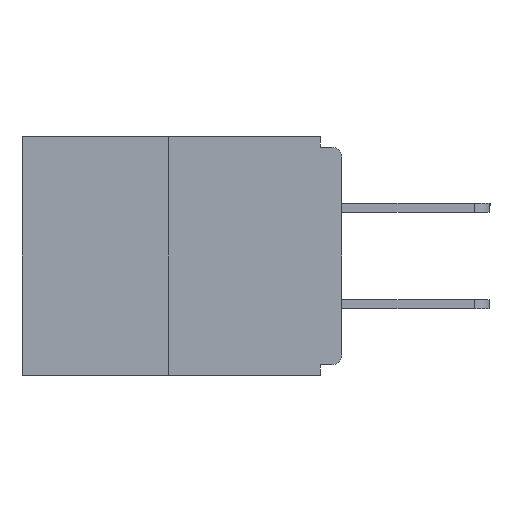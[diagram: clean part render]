
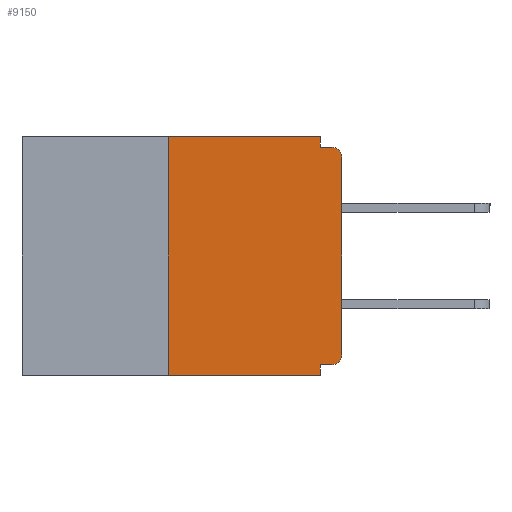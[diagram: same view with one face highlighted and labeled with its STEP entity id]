
A CAD part, left-side view. The second image highlights one B-rep face of the part: STEP entity #9150.
In plain terms, the highlighted planar face has unit normal (-1, 0, 0).
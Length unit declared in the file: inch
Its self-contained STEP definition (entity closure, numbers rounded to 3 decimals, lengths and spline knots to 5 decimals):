
#541 = ORIENTED_EDGE ( 'NONE', *, *, #11632, .F. ) ;
#844 = CARTESIAN_POINT ( 'NONE',  ( 0., 0.25, 0. ) ) ;
#851 = VERTEX_POINT ( 'NONE', #844 ) ;
#1272 = VERTEX_POINT ( 'NONE', #11291 ) ;
#1419 = LINE ( 'NONE', #8853, #1959 ) ;
#1493 = CIRCLE ( 'NONE', #14605, 0.015 ) ;
#1959 = VECTOR ( 'NONE', #2751, 39.37008 ) ;
#2205 = VERTEX_POINT ( 'NONE', #17177 ) ;
#2369 = VECTOR ( 'NONE', #10018, 39.37008 ) ;
#2390 = CARTESIAN_POINT ( 'NONE',  ( 0., 0., 0. ) ) ;
#2751 = DIRECTION ( 'NONE',  ( 0., 0., -1. ) ) ;
#2755 = DIRECTION ( 'NONE',  ( 0., -1., 0. ) ) ;
#2837 = VERTEX_POINT ( 'NONE', #16638 ) ;
#3028 = CARTESIAN_POINT ( 'NONE',  ( 0., 0., -0.015 ) ) ;
#3560 = AXIS2_PLACEMENT_3D ( 'NONE', #7924, #18432, #12229 ) ;
#3826 = DIRECTION ( 'NONE',  ( 0., 0., 1. ) ) ;
#4179 = CIRCLE ( 'NONE', #14873, 0.015 ) ;
#4523 = CARTESIAN_POINT ( 'NONE',  ( 0., 0.031, -0.343 ) ) ;
#5010 = CARTESIAN_POINT ( 'NONE',  ( 0., 0., -0.313 ) ) ;
#5031 = VERTEX_POINT ( 'NONE', #9419 ) ;
#5243 = FACE_OUTER_BOUND ( 'NONE', #17257, .T. ) ;
#5719 = EDGE_CURVE ( 'NONE', #2205, #1272, #18383, .T. ) ;
#5722 = CARTESIAN_POINT ( 'NONE',  ( 0., 0.46, -0.343 ) ) ;
#5821 = CARTESIAN_POINT ( 'NONE',  ( 0., 0.25, 0. ) ) ;
#6054 = LINE ( 'NONE', #4523, #15050 ) ;
#6252 = VERTEX_POINT ( 'NONE', #8470 ) ;
#6328 = EDGE_CURVE ( 'NONE', #12820, #2837, #1419, .T. ) ;
#6375 = CARTESIAN_POINT ( 'NONE',  ( 0., 0.25, -0.343 ) ) ;
#7100 = VECTOR ( 'NONE', #2755, 39.37008 ) ;
#7128 = DIRECTION ( 'NONE',  ( 0., -1., 0. ) ) ;
#7825 = VECTOR ( 'NONE', #7128, 39.37008 ) ;
#7924 = CARTESIAN_POINT ( 'NONE',  ( 0., 0.46, 0. ) ) ;
#8248 = VERTEX_POINT ( 'NONE', #5010 ) ;
#8470 = CARTESIAN_POINT ( 'NONE',  ( 0., 0., -0.03 ) ) ;
#8853 = CARTESIAN_POINT ( 'NONE',  ( 0., 0.031, 0. ) ) ;
#9068 = DIRECTION ( 'NONE',  ( 0., 0., 1. ) ) ;
#9150 = ADVANCED_FACE ( 'NONE', ( #5243 ), #18062, .F. ) ;
#9266 = DIRECTION ( 'NONE',  ( 0., 0., -1. ) ) ;
#9419 = CARTESIAN_POINT ( 'NONE',  ( 0., 0.031, -0.343 ) ) ;
#9457 = VECTOR ( 'NONE', #3826, 39.37008 ) ;
#9468 = EDGE_CURVE ( 'NONE', #2205, #8248, #4179, .T. ) ;
#9645 = LINE ( 'NONE', #2390, #9457 ) ;
#10018 = DIRECTION ( 'NONE',  ( 0., -1., 0. ) ) ;
#10505 = LINE ( 'NONE', #5821, #17161 ) ;
#10525 = ORIENTED_EDGE ( 'NONE', *, *, #15537, .F. ) ;
#10857 = CARTESIAN_POINT ( 'NONE',  ( 0., 0.015, -0.313 ) ) ;
#11016 = DIRECTION ( 'NONE',  ( 0., 1., 0. ) ) ;
#11291 = CARTESIAN_POINT ( 'NONE',  ( 0., 0.031, -0.328 ) ) ;
#11463 = CARTESIAN_POINT ( 'NONE',  ( 0., 0., -0.328 ) ) ;
#11546 = ORIENTED_EDGE ( 'NONE', *, *, #12403, .F. ) ;
#11632 = EDGE_CURVE ( 'NONE', #13246, #851, #10505, .T. ) ;
#11755 = ORIENTED_EDGE ( 'NONE', *, *, #5719, .F. ) ;
#11852 = ORIENTED_EDGE ( 'NONE', *, *, #16260, .T. ) ;
#11929 = EDGE_CURVE ( 'NONE', #851, #12820, #14225, .T. ) ;
#12146 = ORIENTED_EDGE ( 'NONE', *, *, #9468, .T. ) ;
#12229 = DIRECTION ( 'NONE',  ( 0., 0., -1. ) ) ;
#12403 = EDGE_CURVE ( 'NONE', #1272, #5031, #6054, .T. ) ;
#12820 = VERTEX_POINT ( 'NONE', #13845 ) ;
#13246 = VERTEX_POINT ( 'NONE', #6375 ) ;
#13761 = DIRECTION ( 'NONE',  ( -1., 0., 0. ) ) ;
#13845 = CARTESIAN_POINT ( 'NONE',  ( 0., 0.031, 0. ) ) ;
#14225 = LINE ( 'NONE', #17000, #7100 ) ;
#14605 = AXIS2_PLACEMENT_3D ( 'NONE', #17794, #13761, #9266 ) ;
#14842 = EDGE_CURVE ( 'NONE', #6252, #16706, #1493, .T. ) ;
#14873 = AXIS2_PLACEMENT_3D ( 'NONE', #10857, #18501, #15335 ) ;
#15050 = VECTOR ( 'NONE', #16285, 39.37008 ) ;
#15335 = DIRECTION ( 'NONE',  ( 0., 0., -1. ) ) ;
#15369 = VECTOR ( 'NONE', #11016, 39.37008 ) ;
#15537 = EDGE_CURVE ( 'NONE', #2837, #16706, #16117, .T. ) ;
#16117 = LINE ( 'NONE', #3028, #7825 ) ;
#16260 = EDGE_CURVE ( 'NONE', #13246, #5031, #17385, .T. ) ;
#16285 = DIRECTION ( 'NONE',  ( 0., 0., -1. ) ) ;
#16638 = CARTESIAN_POINT ( 'NONE',  ( 0., 0.031, -0.015 ) ) ;
#16706 = VERTEX_POINT ( 'NONE', #17367 ) ;
#16907 = ORIENTED_EDGE ( 'NONE', *, *, #11929, .F. ) ;
#17000 = CARTESIAN_POINT ( 'NONE',  ( 0., 0.46, 0. ) ) ;
#17161 = VECTOR ( 'NONE', #9068, 39.37008 ) ;
#17177 = CARTESIAN_POINT ( 'NONE',  ( 0., 0.015, -0.328 ) ) ;
#17257 = EDGE_LOOP ( 'NONE', ( #16907, #541, #11852, #11546, #11755, #12146, #18770, #17496, #10525, #17485 ) ) ;
#17367 = CARTESIAN_POINT ( 'NONE',  ( 0., 0.015, -0.015 ) ) ;
#17385 = LINE ( 'NONE', #5722, #2369 ) ;
#17485 = ORIENTED_EDGE ( 'NONE', *, *, #6328, .F. ) ;
#17496 = ORIENTED_EDGE ( 'NONE', *, *, #14842, .T. ) ;
#17794 = CARTESIAN_POINT ( 'NONE',  ( 0., 0.015, -0.03 ) ) ;
#18062 = PLANE ( 'NONE',  #3560 ) ;
#18233 = EDGE_CURVE ( 'NONE', #8248, #6252, #9645, .T. ) ;
#18383 = LINE ( 'NONE', #11463, #15369 ) ;
#18432 = DIRECTION ( 'NONE',  ( 1., 0., 0. ) ) ;
#18501 = DIRECTION ( 'NONE',  ( -1., 0., 0. ) ) ;
#18770 = ORIENTED_EDGE ( 'NONE', *, *, #18233, .T. ) ;
